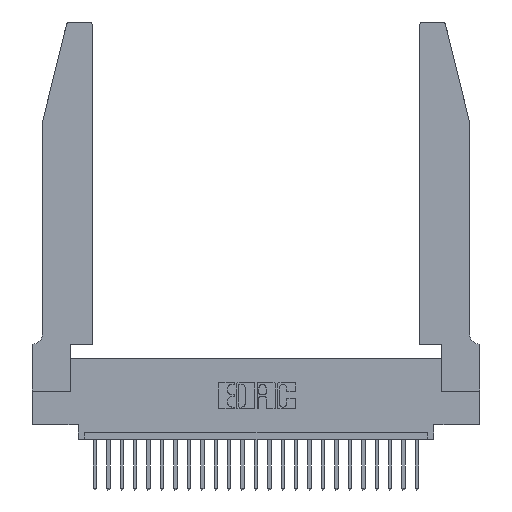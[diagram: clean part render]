
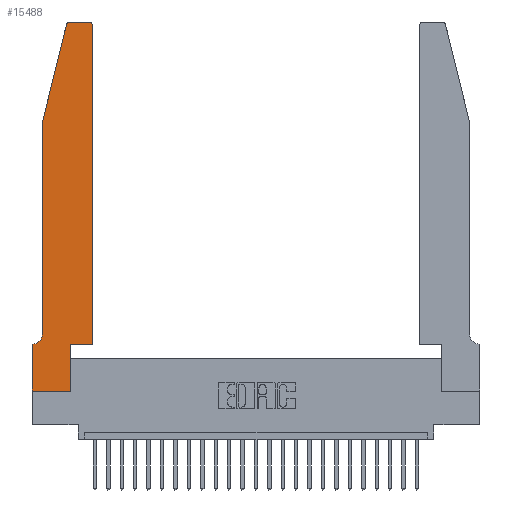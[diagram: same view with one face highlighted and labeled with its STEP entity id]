
A CAD part, top view. The second image highlights one B-rep face of the part: STEP entity #15488.
In plain terms, the highlighted planar face has unit normal (0, 0, 1).
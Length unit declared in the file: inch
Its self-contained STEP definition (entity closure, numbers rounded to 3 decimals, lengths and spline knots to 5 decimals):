
#155 = EDGE_CURVE ( 'NONE', #15642, #6720, #19389, .T. ) ;
#593 = CARTESIAN_POINT ( 'NONE',  ( 0.284, 2.75, 0.37 ) ) ;
#693 = DIRECTION ( 'NONE',  ( 0., 1., 0. ) ) ;
#934 = ORIENTED_EDGE ( 'NONE', *, *, #18837, .T. ) ;
#969 = EDGE_CURVE ( 'NONE', #7705, #8280, #9596, .T. ) ;
#1222 = DIRECTION ( 'NONE',  ( -1., 0., 0. ) ) ;
#1243 = EDGE_CURVE ( 'NONE', #25327, #14056, #23430, .T. ) ;
#1332 = CARTESIAN_POINT ( 'NONE',  ( 0.284, 2.72, 0.37 ) ) ;
#1672 = CARTESIAN_POINT ( 'NONE',  ( 0.25487, 2.72718, 0.37 ) ) ;
#2189 = VECTOR ( 'NONE', #17022, 39.37008 ) ;
#2330 = LINE ( 'NONE', #19175, #18958 ) ;
#3201 = ORIENTED_EDGE ( 'NONE', *, *, #4753, .T. ) ;
#3371 = DIRECTION ( 'NONE',  ( 0., 0., 1. ) ) ;
#3834 = LINE ( 'NONE', #14091, #13890 ) ;
#4165 = EDGE_CURVE ( 'NONE', #14228, #25327, #8768, .T. ) ;
#4400 = LINE ( 'NONE', #12065, #23855 ) ;
#4607 = CARTESIAN_POINT ( 'NONE',  ( 0.4205, 2.75, 0.37 ) ) ;
#4719 = AXIS2_PLACEMENT_3D ( 'NONE', #15721, #19555, #15632 ) ;
#4753 = EDGE_CURVE ( 'NONE', #8280, #17146, #23241, .T. ) ;
#4839 = EDGE_CURVE ( 'NONE', #6720, #14228, #25723, .T. ) ;
#5358 = DIRECTION ( 'NONE',  ( 0., 0., 1. ) ) ;
#5392 = CARTESIAN_POINT ( 'NONE',  ( 0.0755, 0.42, 0.37 ) ) ;
#5713 = CARTESIAN_POINT ( 'NONE',  ( 0.2865, 0.35, 0.37 ) ) ;
#5904 = EDGE_CURVE ( 'NONE', #14056, #11592, #24653, .T. ) ;
#5945 = CARTESIAN_POINT ( 'NONE',  ( 0.0755, 2., 0.37 ) ) ;
#5956 = VECTOR ( 'NONE', #19963, 39.37008 ) ;
#5977 = CARTESIAN_POINT ( 'NONE',  ( 0.4505, 2.72, 0.37 ) ) ;
#6363 = CARTESIAN_POINT ( 'NONE',  ( 0., 0., 0.37 ) ) ;
#6720 = VERTEX_POINT ( 'NONE', #5945 ) ;
#6842 = VERTEX_POINT ( 'NONE', #5977 ) ;
#6915 = ORIENTED_EDGE ( 'NONE', *, *, #155, .T. ) ;
#7207 = DIRECTION ( 'NONE',  ( 1., 0., 0. ) ) ;
#7705 = VERTEX_POINT ( 'NONE', #17109 ) ;
#7960 = EDGE_CURVE ( 'NONE', #6842, #17040, #17342, .T. ) ;
#8280 = VERTEX_POINT ( 'NONE', #15752 ) ;
#8767 = FACE_OUTER_BOUND ( 'NONE', #12419, .T. ) ;
#8768 = CIRCLE ( 'NONE', #4719, 0.07 ) ;
#9241 = CARTESIAN_POINT ( 'NONE',  ( 0., 0., 0.37 ) ) ;
#9325 = ORIENTED_EDGE ( 'NONE', *, *, #11834, .T. ) ;
#9488 = DIRECTION ( 'NONE',  ( 0., 0., 1. ) ) ;
#9546 = VECTOR ( 'NONE', #23914, 39.37008 ) ;
#9596 = LINE ( 'NONE', #5713, #22819 ) ;
#10050 = CARTESIAN_POINT ( 'NONE',  ( 0.4505, 0.35, 0.37 ) ) ;
#10250 = ORIENTED_EDGE ( 'NONE', *, *, #1243, .T. ) ;
#11278 = DIRECTION ( 'NONE',  ( 1., 0., 0. ) ) ;
#11462 = CIRCLE ( 'NONE', #24527, 0.03 ) ;
#11592 = VERTEX_POINT ( 'NONE', #6363 ) ;
#11834 = EDGE_CURVE ( 'NONE', #21311, #15642, #11462, .T. ) ;
#12065 = CARTESIAN_POINT ( 'NONE',  ( 0.4505, 0.35, 0.37 ) ) ;
#12167 = CARTESIAN_POINT ( 'NONE',  ( 0.4505, 0.35, 0.37 ) ) ;
#12406 = DIRECTION ( 'NONE',  ( -1., 0., 0. ) ) ;
#12419 = EDGE_LOOP ( 'NONE', ( #934, #9325, #6915, #24850, #16167, #10250, #14797, #24300, #24381, #3201, #14199, #24866 ) ) ;
#13230 = DIRECTION ( 'NONE',  ( -0.239, -0.971, 0. ) ) ;
#13444 = CARTESIAN_POINT ( 'NONE',  ( 0.4205, 2.72, 0.37 ) ) ;
#13446 = EDGE_CURVE ( 'NONE', #11592, #7705, #2330, .T. ) ;
#13890 = VECTOR ( 'NONE', #12406, 39.37008 ) ;
#14056 = VERTEX_POINT ( 'NONE', #18759 ) ;
#14091 = CARTESIAN_POINT ( 'NONE',  ( 0.2605, 2.75, 0.37 ) ) ;
#14199 = ORIENTED_EDGE ( 'NONE', *, *, #19852, .T. ) ;
#14228 = VERTEX_POINT ( 'NONE', #5392 ) ;
#14797 = ORIENTED_EDGE ( 'NONE', *, *, #5904, .T. ) ;
#15488 = ADVANCED_FACE ( 'NONE', ( #8767 ), #21310, .T. ) ;
#15549 = DIRECTION ( 'NONE',  ( 1., 0., 0. ) ) ;
#15632 = DIRECTION ( 'NONE',  ( -1., 0., 0. ) ) ;
#15642 = VERTEX_POINT ( 'NONE', #1672 ) ;
#15721 = CARTESIAN_POINT ( 'NONE',  ( 0.0055, 0.42, 0.37 ) ) ;
#15752 = CARTESIAN_POINT ( 'NONE',  ( 0.2865, 0.35, 0.37 ) ) ;
#15944 = DIRECTION ( 'NONE',  ( 0., 1., 0. ) ) ;
#16167 = ORIENTED_EDGE ( 'NONE', *, *, #4165, .T. ) ;
#17022 = DIRECTION ( 'NONE',  ( 0., -1., 0. ) ) ;
#17040 = VERTEX_POINT ( 'NONE', #4607 ) ;
#17109 = CARTESIAN_POINT ( 'NONE',  ( 0.2865, 0., 0.37 ) ) ;
#17146 = VERTEX_POINT ( 'NONE', #12167 ) ;
#17342 = CIRCLE ( 'NONE', #17715, 0.03 ) ;
#17715 = AXIS2_PLACEMENT_3D ( 'NONE', #13444, #5358, #15549 ) ;
#18073 = VECTOR ( 'NONE', #1222, 39.37008 ) ;
#18534 = AXIS2_PLACEMENT_3D ( 'NONE', #22602, #9488, #7207 ) ;
#18759 = CARTESIAN_POINT ( 'NONE',  ( 0., 0.35, 0.37 ) ) ;
#18837 = EDGE_CURVE ( 'NONE', #17040, #21311, #3834, .T. ) ;
#18852 = CARTESIAN_POINT ( 'NONE',  ( 0.0755, 0.35, 0.37 ) ) ;
#18856 = CARTESIAN_POINT ( 'NONE',  ( 0.0755, 2., 0.37 ) ) ;
#18958 = VECTOR ( 'NONE', #11278, 39.37008 ) ;
#19175 = CARTESIAN_POINT ( 'NONE',  ( 0., 0., 0.37 ) ) ;
#19389 = LINE ( 'NONE', #25256, #21888 ) ;
#19401 = DIRECTION ( 'NONE',  ( 1., 0., 0. ) ) ;
#19549 = CARTESIAN_POINT ( 'NONE',  ( 0.0055, 0.35, 0.37 ) ) ;
#19555 = DIRECTION ( 'NONE',  ( 0., 0., -1. ) ) ;
#19852 = EDGE_CURVE ( 'NONE', #17146, #6842, #4400, .T. ) ;
#19963 = DIRECTION ( 'NONE',  ( 1., 0., 0. ) ) ;
#21310 = PLANE ( 'NONE',  #18534 ) ;
#21311 = VERTEX_POINT ( 'NONE', #593 ) ;
#21888 = VECTOR ( 'NONE', #13230, 39.37008 ) ;
#22602 = CARTESIAN_POINT ( 'NONE',  ( 0., 0.35, 0.37 ) ) ;
#22819 = VECTOR ( 'NONE', #693, 39.37008 ) ;
#23241 = LINE ( 'NONE', #10050, #5956 ) ;
#23430 = LINE ( 'NONE', #18852, #18073 ) ;
#23855 = VECTOR ( 'NONE', #15944, 39.37008 ) ;
#23914 = DIRECTION ( 'NONE',  ( 0., -1., 0. ) ) ;
#24300 = ORIENTED_EDGE ( 'NONE', *, *, #13446, .T. ) ;
#24381 = ORIENTED_EDGE ( 'NONE', *, *, #969, .T. ) ;
#24527 = AXIS2_PLACEMENT_3D ( 'NONE', #1332, #3371, #19401 ) ;
#24653 = LINE ( 'NONE', #9241, #9546 ) ;
#24850 = ORIENTED_EDGE ( 'NONE', *, *, #4839, .T. ) ;
#24866 = ORIENTED_EDGE ( 'NONE', *, *, #7960, .T. ) ;
#25256 = CARTESIAN_POINT ( 'NONE',  ( 0.0755, 2., 0.37 ) ) ;
#25327 = VERTEX_POINT ( 'NONE', #19549 ) ;
#25723 = LINE ( 'NONE', #18856, #2189 ) ;
